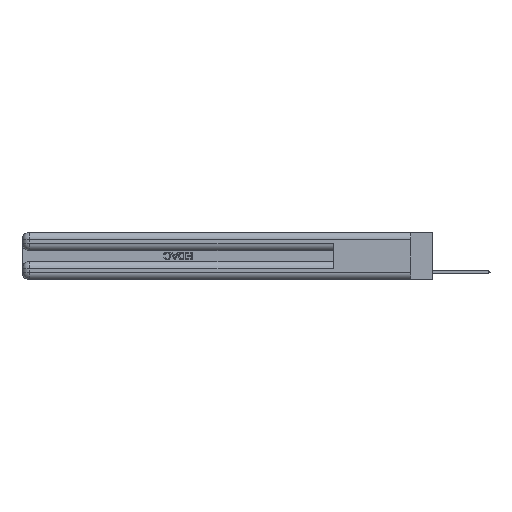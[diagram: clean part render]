
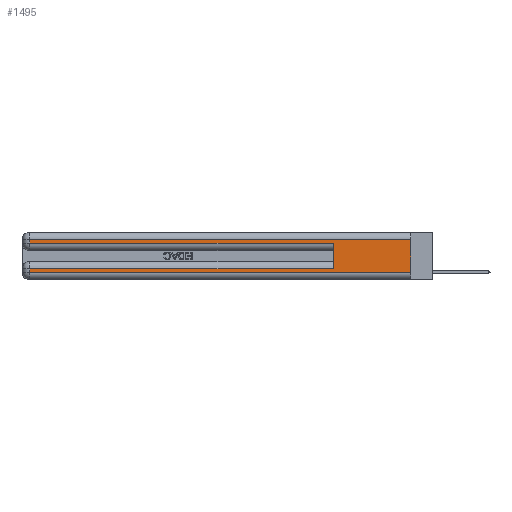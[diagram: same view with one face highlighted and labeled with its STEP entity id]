
A CAD part, left-side view. The second image highlights one B-rep face of the part: STEP entity #1495.
In plain terms, the highlighted planar face has unit normal (-1, 0, 0).
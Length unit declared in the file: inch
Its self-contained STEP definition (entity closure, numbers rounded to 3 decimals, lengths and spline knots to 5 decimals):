
#200 = CARTESIAN_POINT ( 'NONE',  ( 0., 0.6, 0.285 ) ) ;
#944 = EDGE_CURVE ( 'NONE', #1491, #2629, #8800, .T. ) ;
#957 = VECTOR ( 'NONE', #16896, 39.37008 ) ;
#1449 = ORIENTED_EDGE ( 'NONE', *, *, #21440, .T. ) ;
#1491 = VERTEX_POINT ( 'NONE', #21166 ) ;
#1495 = ADVANCED_FACE ( 'NONE', ( #6974 ), #26482, .F. ) ;
#1523 = CARTESIAN_POINT ( 'NONE',  ( 0., 2.94, 0.285 ) ) ;
#2337 = EDGE_CURVE ( 'NONE', #23590, #16549, #31501, .T. ) ;
#2511 = EDGE_CURVE ( 'NONE', #28031, #21987, #20062, .T. ) ;
#2629 = VERTEX_POINT ( 'NONE', #1523 ) ;
#3658 = DIRECTION ( 'NONE',  ( 0., 0., -1. ) ) ;
#3745 = EDGE_CURVE ( 'NONE', #28031, #1491, #29618, .T. ) ;
#3753 = CARTESIAN_POINT ( 'NONE',  ( 0., 2.94, 0.06 ) ) ;
#4109 = ORIENTED_EDGE ( 'NONE', *, *, #22167, .T. ) ;
#4118 = DIRECTION ( 'NONE',  ( 0., -1., 0. ) ) ;
#4717 = DIRECTION ( 'NONE',  ( 1., 0., 0. ) ) ;
#4865 = VERTEX_POINT ( 'NONE', #7137 ) ;
#5372 = VECTOR ( 'NONE', #26678, 39.37008 ) ;
#5778 = CARTESIAN_POINT ( 'NONE',  ( 0., 0., 0.31 ) ) ;
#6819 = ORIENTED_EDGE ( 'NONE', *, *, #944, .T. ) ;
#6974 = FACE_OUTER_BOUND ( 'NONE', #30506, .T. ) ;
#7047 = VECTOR ( 'NONE', #4118, 39.37008 ) ;
#7137 = CARTESIAN_POINT ( 'NONE',  ( 0., 2.94, 0.085 ) ) ;
#7695 = DIRECTION ( 'NONE',  ( 0., -1., 0. ) ) ;
#7776 = DIRECTION ( 'NONE',  ( 0., 1., 0. ) ) ;
#8800 = LINE ( 'NONE', #16205, #9877 ) ;
#9572 = CARTESIAN_POINT ( 'NONE',  ( 0., 0., 0.06 ) ) ;
#9877 = VECTOR ( 'NONE', #26031, 39.37008 ) ;
#10200 = LINE ( 'NONE', #29844, #23553 ) ;
#12216 = LINE ( 'NONE', #29610, #23679 ) ;
#13152 = VECTOR ( 'NONE', #19751, 39.37008 ) ;
#14636 = CARTESIAN_POINT ( 'NONE',  ( 0., 0., 0.31 ) ) ;
#15916 = LINE ( 'NONE', #25745, #28721 ) ;
#16205 = CARTESIAN_POINT ( 'NONE',  ( 0., 2.94, 0.37 ) ) ;
#16549 = VERTEX_POINT ( 'NONE', #200 ) ;
#16638 = ORIENTED_EDGE ( 'NONE', *, *, #3745, .T. ) ;
#16759 = ORIENTED_EDGE ( 'NONE', *, *, #26581, .T. ) ;
#16846 = CARTESIAN_POINT ( 'NONE',  ( 0., 0.6, 0.145 ) ) ;
#16896 = DIRECTION ( 'NONE',  ( 0., 1., 0. ) ) ;
#17374 = ORIENTED_EDGE ( 'NONE', *, *, #2337, .F. ) ;
#18331 = EDGE_CURVE ( 'NONE', #4865, #23242, #15916, .T. ) ;
#19751 = DIRECTION ( 'NONE',  ( 0., 0., -1. ) ) ;
#20062 = LINE ( 'NONE', #29887, #13152 ) ;
#21166 = CARTESIAN_POINT ( 'NONE',  ( 0., 2.94, 0.31 ) ) ;
#21204 = LINE ( 'NONE', #23456, #7047 ) ;
#21440 = EDGE_CURVE ( 'NONE', #23242, #21987, #21204, .T. ) ;
#21987 = VERTEX_POINT ( 'NONE', #9572 ) ;
#22167 = EDGE_CURVE ( 'NONE', #23590, #4865, #10200, .T. ) ;
#23242 = VERTEX_POINT ( 'NONE', #3753 ) ;
#23456 = CARTESIAN_POINT ( 'NONE',  ( 0., 0., 0.06 ) ) ;
#23553 = VECTOR ( 'NONE', #7776, 39.37008 ) ;
#23590 = VERTEX_POINT ( 'NONE', #30301 ) ;
#23679 = VECTOR ( 'NONE', #7695, 39.37008 ) ;
#23734 = DIRECTION ( 'NONE',  ( 0., 0., -1. ) ) ;
#23822 = AXIS2_PLACEMENT_3D ( 'NONE', #31293, #4717, #23734 ) ;
#25745 = CARTESIAN_POINT ( 'NONE',  ( 0., 2.94, 0.37 ) ) ;
#25858 = ORIENTED_EDGE ( 'NONE', *, *, #18331, .T. ) ;
#26031 = DIRECTION ( 'NONE',  ( 0., 0., -1. ) ) ;
#26482 = PLANE ( 'NONE',  #23822 ) ;
#26581 = EDGE_CURVE ( 'NONE', #2629, #16549, #12216, .T. ) ;
#26678 = DIRECTION ( 'NONE',  ( 0., 0., 1. ) ) ;
#28031 = VERTEX_POINT ( 'NONE', #5778 ) ;
#28495 = ORIENTED_EDGE ( 'NONE', *, *, #2511, .F. ) ;
#28721 = VECTOR ( 'NONE', #3658, 39.37008 ) ;
#29610 = CARTESIAN_POINT ( 'NONE',  ( 0., 0., 0.285 ) ) ;
#29618 = LINE ( 'NONE', #14636, #957 ) ;
#29844 = CARTESIAN_POINT ( 'NONE',  ( 0., 0., 0.085 ) ) ;
#29887 = CARTESIAN_POINT ( 'NONE',  ( 0., 0., 0.37 ) ) ;
#30301 = CARTESIAN_POINT ( 'NONE',  ( 0., 0.6, 0.085 ) ) ;
#30506 = EDGE_LOOP ( 'NONE', ( #28495, #16638, #6819, #16759, #17374, #4109, #25858, #1449 ) ) ;
#31293 = CARTESIAN_POINT ( 'NONE',  ( 0., 0., 0.37 ) ) ;
#31501 = LINE ( 'NONE', #16846, #5372 ) ;
